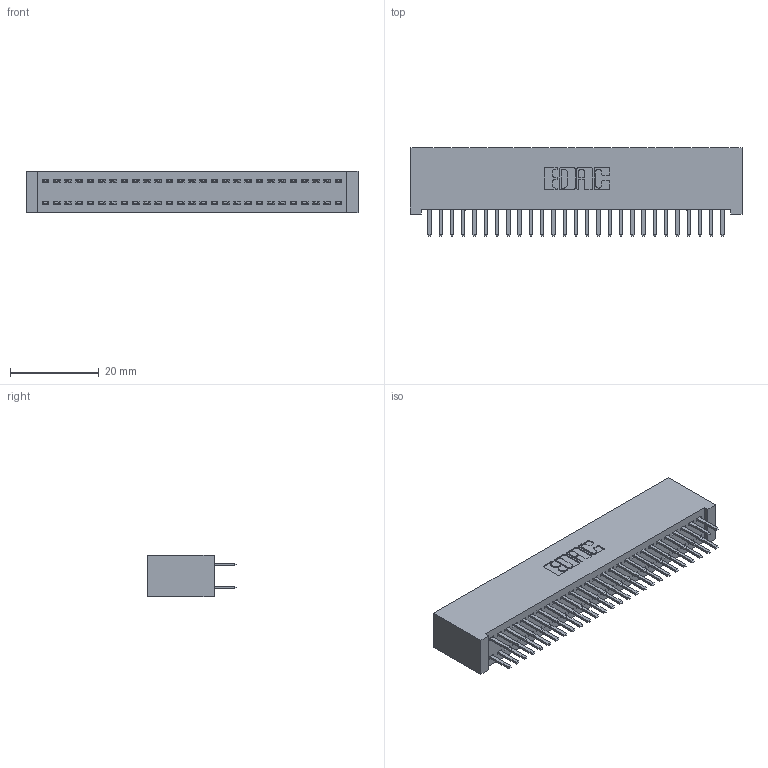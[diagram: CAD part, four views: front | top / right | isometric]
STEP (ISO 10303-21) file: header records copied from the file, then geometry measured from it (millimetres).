
FILE_DESCRIPTION (( 'STEP AP203' ), '1' );
FILE_NAME ('342-054-520-201.STEP', '2018-08-12T23:42:55', ( '' ), ( '' ), 'SwSTEP 2.0', 'SolidWorks 2016', '' );
FILE_SCHEMA (( 'CONFIG_CONTROL_DESIGN' ));
Length unit declared in the file: inch
Products named in the file (3): 342 Part_Lugless; 345-292-001_345-293-120; 342-054-520-201
Assembly tree (55 placements, depth 2):
  342-054-520-201
    342 Part_Lugless
    345-292-001_345-293-120  x54
Bounding box: 74.83 x 20.02 x 9.4 mm (x, y, z)
Volume: 7068.1 mm3; surface area: 11525.7 mm2
Topology: 55 solids, 55 shells, 3126 faces, 9077 edges, 5906 vertices
Faces by surface type: plane 2114, cylinder 1012
Entity records: 19015 total; most frequent: CARTESIAN_POINT 3178, ORIENTED_EDGE 3102, DIRECTION 2723, EDGE_CURVE 1551, LINE 1427, VECTOR 1427, VERTEX_POINT 1030, AXIS2_PLACEMENT_3D 648
